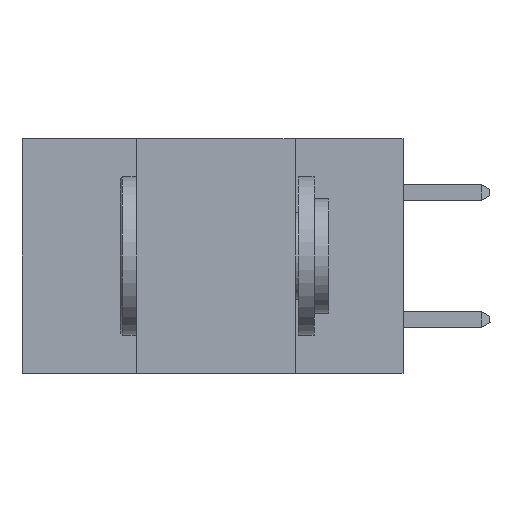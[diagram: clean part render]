
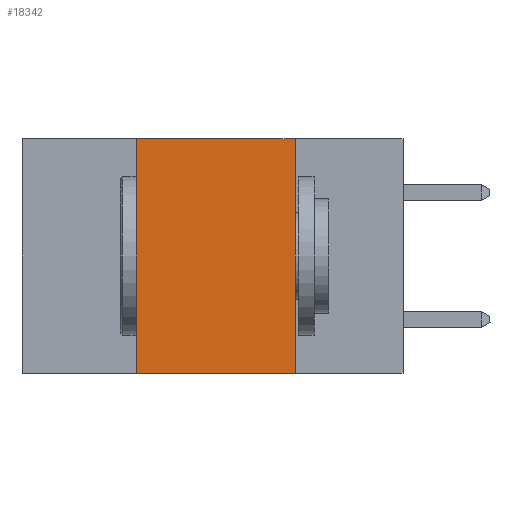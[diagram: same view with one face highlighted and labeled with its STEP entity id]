
A CAD part, left-side view. The second image highlights one B-rep face of the part: STEP entity #18342.
In plain terms, the highlighted planar face has unit normal (-1, 0, 0).
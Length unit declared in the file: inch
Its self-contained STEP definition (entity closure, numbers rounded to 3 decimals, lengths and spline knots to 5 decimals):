
#978 = LINE ( 'NONE', #7156, #5216 ) ;
#2565 = DIRECTION ( 'NONE',  ( 0., 0., -1. ) ) ;
#2658 = VECTOR ( 'NONE', #7666, 39.37008 ) ;
#2875 = FACE_OUTER_BOUND ( 'NONE', #15053, .T. ) ;
#2913 = VERTEX_POINT ( 'NONE', #4751 ) ;
#3596 = LINE ( 'NONE', #16091, #16970 ) ;
#4751 = CARTESIAN_POINT ( 'NONE',  ( 0., 0.42, 0. ) ) ;
#5216 = VECTOR ( 'NONE', #8875, 39.37008 ) ;
#5929 = CARTESIAN_POINT ( 'NONE',  ( 0., 0.6, -0.37 ) ) ;
#6573 = VERTEX_POINT ( 'NONE', #11604 ) ;
#7042 = CARTESIAN_POINT ( 'NONE',  ( 0., 0.42, -0.37 ) ) ;
#7156 = CARTESIAN_POINT ( 'NONE',  ( 0., 0.17, 0. ) ) ;
#7666 = DIRECTION ( 'NONE',  ( 0., -1., 0. ) ) ;
#8062 = VERTEX_POINT ( 'NONE', #12383 ) ;
#8520 = LINE ( 'NONE', #13907, #21781 ) ;
#8875 = DIRECTION ( 'NONE',  ( 0., 0., -1. ) ) ;
#9320 = EDGE_CURVE ( 'NONE', #6573, #8062, #978, .T. ) ;
#9543 = AXIS2_PLACEMENT_3D ( 'NONE', #11295, #13073, #2565 ) ;
#9935 = VERTEX_POINT ( 'NONE', #7042 ) ;
#11053 = ORIENTED_EDGE ( 'NONE', *, *, #16830, .T. ) ;
#11295 = CARTESIAN_POINT ( 'NONE',  ( 0., 0.6, 0. ) ) ;
#11604 = CARTESIAN_POINT ( 'NONE',  ( 0., 0.17, 0. ) ) ;
#12383 = CARTESIAN_POINT ( 'NONE',  ( 0., 0.17, -0.37 ) ) ;
#13073 = DIRECTION ( 'NONE',  ( 1., 0., 0. ) ) ;
#13907 = CARTESIAN_POINT ( 'NONE',  ( 0., 0.6, 0. ) ) ;
#14903 = ORIENTED_EDGE ( 'NONE', *, *, #19932, .F. ) ;
#15053 = EDGE_LOOP ( 'NONE', ( #15177, #14903, #19433, #11053 ) ) ;
#15177 = ORIENTED_EDGE ( 'NONE', *, *, #9320, .F. ) ;
#15695 = DIRECTION ( 'NONE',  ( 0., -1., 0. ) ) ;
#16091 = CARTESIAN_POINT ( 'NONE',  ( 0., 0.42, 0. ) ) ;
#16830 = EDGE_CURVE ( 'NONE', #9935, #8062, #21145, .T. ) ;
#16970 = VECTOR ( 'NONE', #17814, 39.37008 ) ;
#17814 = DIRECTION ( 'NONE',  ( 0., 0., 1. ) ) ;
#18342 = ADVANCED_FACE ( 'NONE', ( #2875 ), #21611, .F. ) ;
#19433 = ORIENTED_EDGE ( 'NONE', *, *, #21058, .F. ) ;
#19932 = EDGE_CURVE ( 'NONE', #2913, #6573, #8520, .T. ) ;
#21058 = EDGE_CURVE ( 'NONE', #9935, #2913, #3596, .T. ) ;
#21145 = LINE ( 'NONE', #5929, #2658 ) ;
#21611 = PLANE ( 'NONE',  #9543 ) ;
#21781 = VECTOR ( 'NONE', #15695, 39.37008 ) ;
